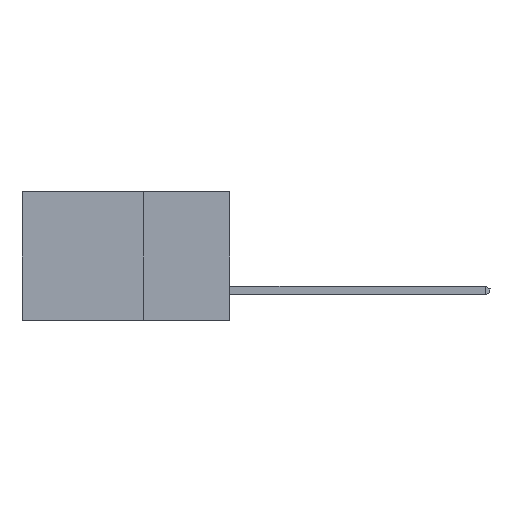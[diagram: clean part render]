
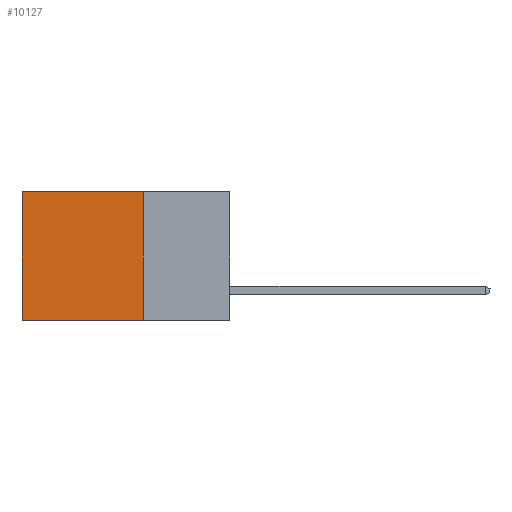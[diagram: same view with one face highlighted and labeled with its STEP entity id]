
A CAD part, left-side view. The second image highlights one B-rep face of the part: STEP entity #10127.
In plain terms, the highlighted planar face has unit normal (-1, 0, 0).
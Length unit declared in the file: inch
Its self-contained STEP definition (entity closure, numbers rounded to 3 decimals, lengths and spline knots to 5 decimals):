
#110 = CARTESIAN_POINT ( 'NONE',  ( 0.2615, 0.6, -0.37 ) ) ;
#798 = FACE_OUTER_BOUND ( 'NONE', #9543, .T. ) ;
#986 = CARTESIAN_POINT ( 'NONE',  ( 0.2615, 0.25, -0.37 ) ) ;
#1149 = AXIS2_PLACEMENT_3D ( 'NONE', #986, #9590, #7670 ) ;
#1374 = DIRECTION ( 'NONE',  ( 0., 1., 0. ) ) ;
#1658 = EDGE_CURVE ( 'NONE', #7900, #11402, #8499, .T. ) ;
#1669 = CARTESIAN_POINT ( 'NONE',  ( 0.2615, 0.6, -0.37 ) ) ;
#1893 = CARTESIAN_POINT ( 'NONE',  ( 0.2615, 0.25, -0.37 ) ) ;
#2269 = CARTESIAN_POINT ( 'NONE',  ( 0.2615, 0.25, -0.37 ) ) ;
#2320 = DIRECTION ( 'NONE',  ( 0., 1., 0. ) ) ;
#2335 = LINE ( 'NONE', #2269, #2756 ) ;
#2381 = CARTESIAN_POINT ( 'NONE',  ( 0.2615, 0.25, 0. ) ) ;
#2756 = VECTOR ( 'NONE', #11082, 39.37008 ) ;
#3576 = ORIENTED_EDGE ( 'NONE', *, *, #11277, .F. ) ;
#5590 = PLANE ( 'NONE',  #1149 ) ;
#5615 = VERTEX_POINT ( 'NONE', #1893 ) ;
#6674 = CARTESIAN_POINT ( 'NONE',  ( 0.2615, 0.6, 0. ) ) ;
#7564 = ORIENTED_EDGE ( 'NONE', *, *, #8935, .F. ) ;
#7670 = DIRECTION ( 'NONE',  ( 0., 0., -1. ) ) ;
#7900 = VERTEX_POINT ( 'NONE', #6674 ) ;
#8031 = EDGE_CURVE ( 'NONE', #8929, #7900, #8071, .T. ) ;
#8071 = LINE ( 'NONE', #2381, #10228 ) ;
#8140 = VECTOR ( 'NONE', #1374, 39.37008 ) ;
#8499 = LINE ( 'NONE', #1669, #12380 ) ;
#8929 = VERTEX_POINT ( 'NONE', #9116 ) ;
#8935 = EDGE_CURVE ( 'NONE', #8929, #5615, #2335, .T. ) ;
#9116 = CARTESIAN_POINT ( 'NONE',  ( 0.2615, 0.25, 0. ) ) ;
#9543 = EDGE_LOOP ( 'NONE', ( #12230, #3576, #7564, #11223 ) ) ;
#9590 = DIRECTION ( 'NONE',  ( 1., 0., 0. ) ) ;
#10127 = ADVANCED_FACE ( 'NONE', ( #798 ), #5590, .F. ) ;
#10228 = VECTOR ( 'NONE', #2320, 39.37008 ) ;
#11082 = DIRECTION ( 'NONE',  ( 0., 0., -1. ) ) ;
#11223 = ORIENTED_EDGE ( 'NONE', *, *, #8031, .T. ) ;
#11277 = EDGE_CURVE ( 'NONE', #5615, #11402, #12078, .T. ) ;
#11402 = VERTEX_POINT ( 'NONE', #110 ) ;
#11488 = DIRECTION ( 'NONE',  ( 0., 0., -1. ) ) ;
#11949 = CARTESIAN_POINT ( 'NONE',  ( 0.2615, 0.25, -0.37 ) ) ;
#12078 = LINE ( 'NONE', #11949, #8140 ) ;
#12230 = ORIENTED_EDGE ( 'NONE', *, *, #1658, .T. ) ;
#12380 = VECTOR ( 'NONE', #11488, 39.37008 ) ;
